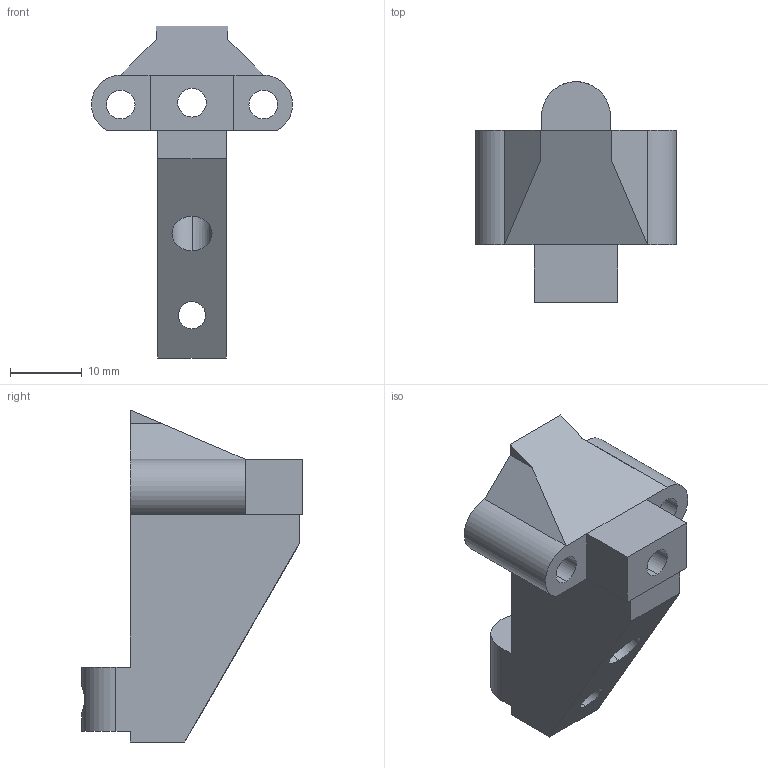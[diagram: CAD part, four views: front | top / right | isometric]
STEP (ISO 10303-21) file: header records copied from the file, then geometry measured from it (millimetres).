
FILE_DESCRIPTION (( 'STEP AP203' ), '1' );
FILE_NAME ('PistolGripAdapter.STEP', '2019-09-03T07:04:50', ( '' ), ( '' ), 'SwSTEP 2.0', 'SolidWorks 2018', '' );
FILE_SCHEMA (( 'CONFIG_CONTROL_DESIGN' ));
Length unit declared in the file: millimetre
Products named in the file (1): PistolGripAdapter
Bounding box: 28.04 x 30.8 x 46.29 mm (x, y, z)
Volume: 8988 mm3; surface area: 4793.3 mm2
Topology: 1 solids, 1 shells, 34 faces, 94 edges, 62 vertices
Faces by surface type: plane 21, cylinder 13
Entity records: 1233 total; most frequent: CARTESIAN_POINT 261, ORIENTED_EDGE 188, DIRECTION 178, EDGE_CURVE 94, VECTOR 68, LINE 68, VERTEX_POINT 62, AXIS2_PLACEMENT_3D 55
